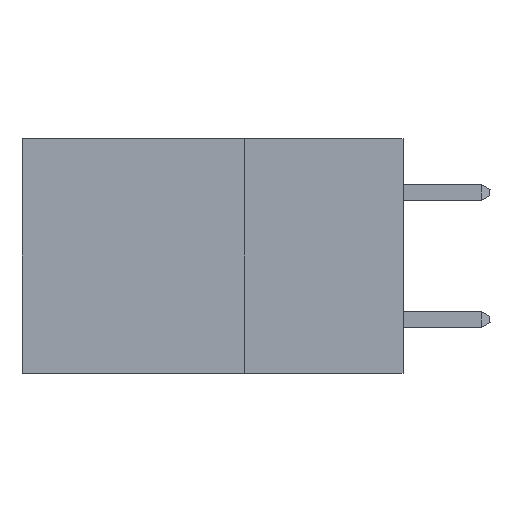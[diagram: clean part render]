
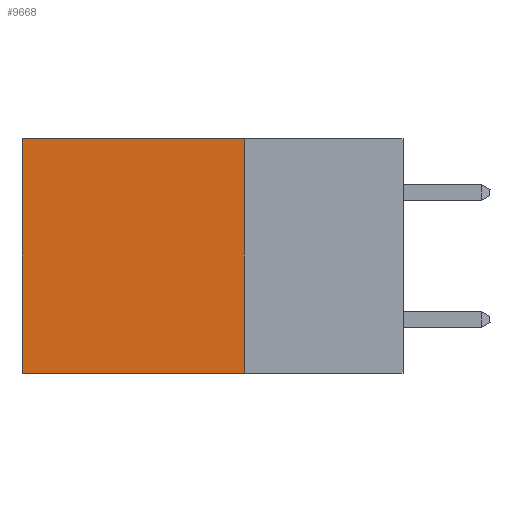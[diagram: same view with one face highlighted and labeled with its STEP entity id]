
A CAD part, left-side view. The second image highlights one B-rep face of the part: STEP entity #9668.
In plain terms, the highlighted planar face has unit normal (-1, 0, 0).
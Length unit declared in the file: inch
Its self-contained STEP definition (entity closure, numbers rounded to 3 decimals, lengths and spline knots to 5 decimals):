
#640 = LINE ( 'NONE', #8406, #5143 ) ;
#1356 = CARTESIAN_POINT ( 'NONE',  ( 0.2875, 0.6, 0. ) ) ;
#2119 = EDGE_LOOP ( 'NONE', ( #3300, #5224, #2217, #5195 ) ) ;
#2217 = ORIENTED_EDGE ( 'NONE', *, *, #7213, .F. ) ;
#2368 = FACE_OUTER_BOUND ( 'NONE', #2119, .T. ) ;
#2371 = CARTESIAN_POINT ( 'NONE',  ( 0.2875, 0.25, -0.37 ) ) ;
#2392 = LINE ( 'NONE', #2791, #6409 ) ;
#2429 = LINE ( 'NONE', #6968, #8900 ) ;
#2662 = DIRECTION ( 'NONE',  ( 0., 1., 0. ) ) ;
#2791 = CARTESIAN_POINT ( 'NONE',  ( 0.2875, 0.6, 0. ) ) ;
#3300 = ORIENTED_EDGE ( 'NONE', *, *, #8791, .T. ) ;
#3307 = DIRECTION ( 'NONE',  ( 0., 0., -1. ) ) ;
#3932 = EDGE_CURVE ( 'NONE', #5859, #8039, #2429, .T. ) ;
#4272 = CARTESIAN_POINT ( 'NONE',  ( 0.2875, 0.25, 0. ) ) ;
#4693 = LINE ( 'NONE', #4272, #5506 ) ;
#5097 = EDGE_CURVE ( 'NONE', #7131, #8218, #640, .T. ) ;
#5143 = VECTOR ( 'NONE', #5869, 39.37008 ) ;
#5195 = ORIENTED_EDGE ( 'NONE', *, *, #5097, .T. ) ;
#5224 = ORIENTED_EDGE ( 'NONE', *, *, #3932, .F. ) ;
#5506 = VECTOR ( 'NONE', #10076, 39.37008 ) ;
#5554 = AXIS2_PLACEMENT_3D ( 'NONE', #6717, #8390, #3307 ) ;
#5859 = VERTEX_POINT ( 'NONE', #2371 ) ;
#5869 = DIRECTION ( 'NONE',  ( 0., 1., 0. ) ) ;
#6239 = DIRECTION ( 'NONE',  ( 0., 0., -1. ) ) ;
#6409 = VECTOR ( 'NONE', #6239, 39.37008 ) ;
#6717 = CARTESIAN_POINT ( 'NONE',  ( 0.2875, 0.25, 0. ) ) ;
#6968 = CARTESIAN_POINT ( 'NONE',  ( 0.2875, 0.25, -0.37 ) ) ;
#7131 = VERTEX_POINT ( 'NONE', #9968 ) ;
#7213 = EDGE_CURVE ( 'NONE', #7131, #5859, #4693, .T. ) ;
#7566 = PLANE ( 'NONE',  #5554 ) ;
#8039 = VERTEX_POINT ( 'NONE', #8698 ) ;
#8218 = VERTEX_POINT ( 'NONE', #1356 ) ;
#8390 = DIRECTION ( 'NONE',  ( 1., 0., 0. ) ) ;
#8406 = CARTESIAN_POINT ( 'NONE',  ( 0.2875, 0.25, 0. ) ) ;
#8698 = CARTESIAN_POINT ( 'NONE',  ( 0.2875, 0.6, -0.37 ) ) ;
#8791 = EDGE_CURVE ( 'NONE', #8218, #8039, #2392, .T. ) ;
#8900 = VECTOR ( 'NONE', #2662, 39.37008 ) ;
#9668 = ADVANCED_FACE ( 'NONE', ( #2368 ), #7566, .F. ) ;
#9968 = CARTESIAN_POINT ( 'NONE',  ( 0.2875, 0.25, 0. ) ) ;
#10076 = DIRECTION ( 'NONE',  ( 0., 0., -1. ) ) ;
